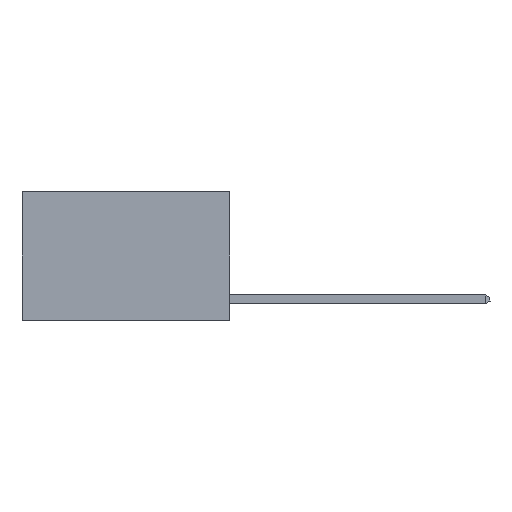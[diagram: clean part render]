
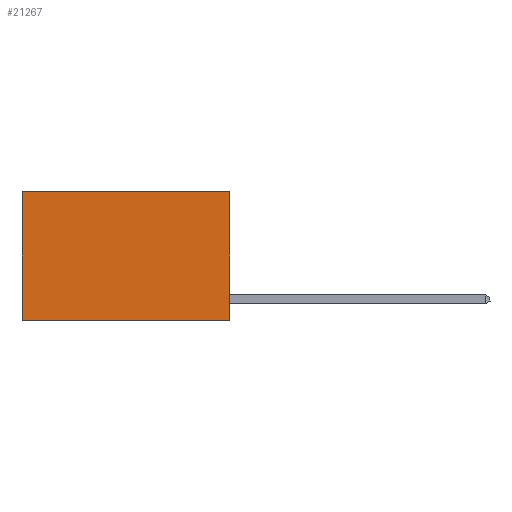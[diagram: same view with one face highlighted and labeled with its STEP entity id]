
A CAD part, left-side view. The second image highlights one B-rep face of the part: STEP entity #21267.
In plain terms, the highlighted planar face has unit normal (-1, 0, 0).
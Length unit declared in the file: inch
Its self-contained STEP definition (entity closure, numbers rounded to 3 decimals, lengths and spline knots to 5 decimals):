
#287 = CARTESIAN_POINT ( 'NONE',  ( 0.2625, 0.6, -0.37 ) ) ;
#1163 = AXIS2_PLACEMENT_3D ( 'NONE', #18432, #14990, #18354 ) ;
#2021 = DIRECTION ( 'NONE',  ( 0., 0., -1. ) ) ;
#2175 = VECTOR ( 'NONE', #6522, 39.37008 ) ;
#3190 = CARTESIAN_POINT ( 'NONE',  ( 0.2625, 0., 0. ) ) ;
#3694 = DIRECTION ( 'NONE',  ( 0., 1., 0. ) ) ;
#3808 = EDGE_CURVE ( 'NONE', #12324, #6855, #20295, .T. ) ;
#4098 = VERTEX_POINT ( 'NONE', #9817 ) ;
#6237 = ORIENTED_EDGE ( 'NONE', *, *, #3808, .T. ) ;
#6522 = DIRECTION ( 'NONE',  ( 0., 0., -1. ) ) ;
#6855 = VERTEX_POINT ( 'NONE', #287 ) ;
#7476 = EDGE_CURVE ( 'NONE', #17822, #12324, #11713, .T. ) ;
#7709 = VECTOR ( 'NONE', #2021, 39.37008 ) ;
#8323 = ORIENTED_EDGE ( 'NONE', *, *, #7476, .T. ) ;
#8398 = EDGE_CURVE ( 'NONE', #4098, #6855, #10357, .T. ) ;
#9168 = ORIENTED_EDGE ( 'NONE', *, *, #8398, .F. ) ;
#9817 = CARTESIAN_POINT ( 'NONE',  ( 0.2625, 0., -0.37 ) ) ;
#10085 = CARTESIAN_POINT ( 'NONE',  ( 0.2625, 0., 0. ) ) ;
#10357 = LINE ( 'NONE', #20862, #19008 ) ;
#10928 = VECTOR ( 'NONE', #15119, 39.37008 ) ;
#11713 = LINE ( 'NONE', #10085, #10928 ) ;
#12282 = CARTESIAN_POINT ( 'NONE',  ( 0.2625, 0., 0. ) ) ;
#12324 = VERTEX_POINT ( 'NONE', #16856 ) ;
#13868 = EDGE_CURVE ( 'NONE', #17822, #4098, #19303, .T. ) ;
#14990 = DIRECTION ( 'NONE',  ( 1., 0., 0. ) ) ;
#15119 = DIRECTION ( 'NONE',  ( 0., 1., 0. ) ) ;
#15159 = CARTESIAN_POINT ( 'NONE',  ( 0.2625, 0.6, 0. ) ) ;
#16856 = CARTESIAN_POINT ( 'NONE',  ( 0.2625, 0.6, 0. ) ) ;
#17477 = FACE_OUTER_BOUND ( 'NONE', #18179, .T. ) ;
#17822 = VERTEX_POINT ( 'NONE', #3190 ) ;
#18179 = EDGE_LOOP ( 'NONE', ( #6237, #9168, #21192, #8323 ) ) ;
#18354 = DIRECTION ( 'NONE',  ( 0., 0., -1. ) ) ;
#18432 = CARTESIAN_POINT ( 'NONE',  ( 0.2625, 0., 0. ) ) ;
#19008 = VECTOR ( 'NONE', #3694, 39.37008 ) ;
#19303 = LINE ( 'NONE', #12282, #7709 ) ;
#20295 = LINE ( 'NONE', #15159, #2175 ) ;
#20862 = CARTESIAN_POINT ( 'NONE',  ( 0.2625, 0., -0.37 ) ) ;
#21192 = ORIENTED_EDGE ( 'NONE', *, *, #13868, .F. ) ;
#21267 = ADVANCED_FACE ( 'NONE', ( #17477 ), #21668, .F. ) ;
#21668 = PLANE ( 'NONE',  #1163 ) ;
